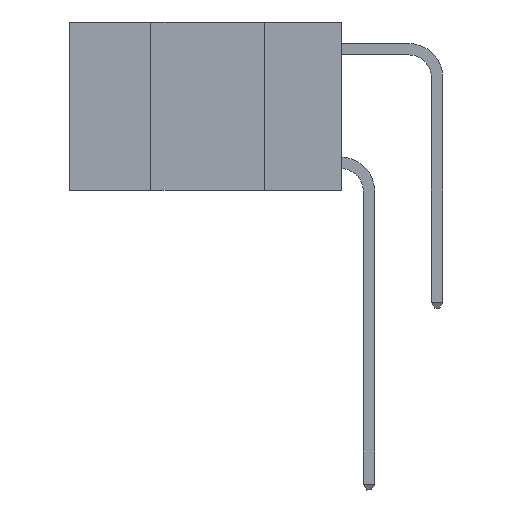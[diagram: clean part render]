
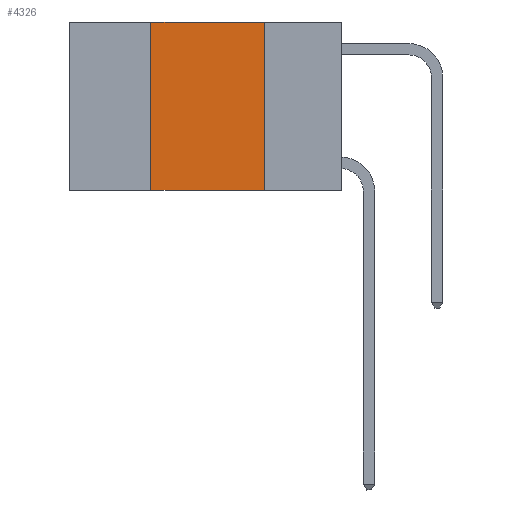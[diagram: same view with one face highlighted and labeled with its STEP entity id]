
A CAD part, left-side view. The second image highlights one B-rep face of the part: STEP entity #4326.
In plain terms, the highlighted planar face has unit normal (-1, 0, 0).
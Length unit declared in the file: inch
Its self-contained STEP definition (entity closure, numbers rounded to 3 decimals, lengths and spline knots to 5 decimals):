
#132 = CARTESIAN_POINT ( 'NONE',  ( 0., 0.17, 0. ) ) ;
#504 = ORIENTED_EDGE ( 'NONE', *, *, #12660, .F. ) ;
#914 = LINE ( 'NONE', #14312, #15231 ) ;
#1157 = VECTOR ( 'NONE', #8865, 39.37008 ) ;
#2528 = DIRECTION ( 'NONE',  ( 0., -1., 0. ) ) ;
#3025 = CARTESIAN_POINT ( 'NONE',  ( 0., 0.17, 0. ) ) ;
#3976 = VECTOR ( 'NONE', #14427, 39.37008 ) ;
#4326 = ADVANCED_FACE ( 'NONE', ( #6531 ), #18191, .F. ) ;
#5093 = CARTESIAN_POINT ( 'NONE',  ( 0., 0.6, 0. ) ) ;
#5194 = ORIENTED_EDGE ( 'NONE', *, *, #11123, .F. ) ;
#5197 = VECTOR ( 'NONE', #18385, 39.37008 ) ;
#5500 = ORIENTED_EDGE ( 'NONE', *, *, #10942, .F. ) ;
#5713 = LINE ( 'NONE', #3025, #1157 ) ;
#6531 = FACE_OUTER_BOUND ( 'NONE', #12290, .T. ) ;
#7009 = VERTEX_POINT ( 'NONE', #9538 ) ;
#7562 = VERTEX_POINT ( 'NONE', #8433 ) ;
#7977 = VERTEX_POINT ( 'NONE', #8300 ) ;
#8232 = ORIENTED_EDGE ( 'NONE', *, *, #18618, .T. ) ;
#8300 = CARTESIAN_POINT ( 'NONE',  ( 0., 0.42, 0. ) ) ;
#8433 = CARTESIAN_POINT ( 'NONE',  ( 0., 0.42, -0.37 ) ) ;
#8865 = DIRECTION ( 'NONE',  ( 0., 0., -1. ) ) ;
#9500 = DIRECTION ( 'NONE',  ( 0., 0., -1. ) ) ;
#9538 = CARTESIAN_POINT ( 'NONE',  ( 0., 0.17, -0.37 ) ) ;
#10942 = EDGE_CURVE ( 'NONE', #14234, #7009, #5713, .T. ) ;
#11123 = EDGE_CURVE ( 'NONE', #7977, #14234, #914, .T. ) ;
#11292 = LINE ( 'NONE', #14107, #5197 ) ;
#12290 = EDGE_LOOP ( 'NONE', ( #5500, #5194, #504, #8232 ) ) ;
#12660 = EDGE_CURVE ( 'NONE', #7562, #7977, #11292, .T. ) ;
#13057 = LINE ( 'NONE', #14711, #3976 ) ;
#14107 = CARTESIAN_POINT ( 'NONE',  ( 0., 0.42, 0. ) ) ;
#14234 = VERTEX_POINT ( 'NONE', #132 ) ;
#14312 = CARTESIAN_POINT ( 'NONE',  ( 0., 0.6, 0. ) ) ;
#14427 = DIRECTION ( 'NONE',  ( 0., -1., 0. ) ) ;
#14711 = CARTESIAN_POINT ( 'NONE',  ( 0., 0.6, -0.37 ) ) ;
#14800 = AXIS2_PLACEMENT_3D ( 'NONE', #5093, #16785, #9500 ) ;
#15231 = VECTOR ( 'NONE', #2528, 39.37008 ) ;
#16785 = DIRECTION ( 'NONE',  ( 1., 0., 0. ) ) ;
#18191 = PLANE ( 'NONE',  #14800 ) ;
#18385 = DIRECTION ( 'NONE',  ( 0., 0., 1. ) ) ;
#18618 = EDGE_CURVE ( 'NONE', #7562, #7009, #13057, .T. ) ;
